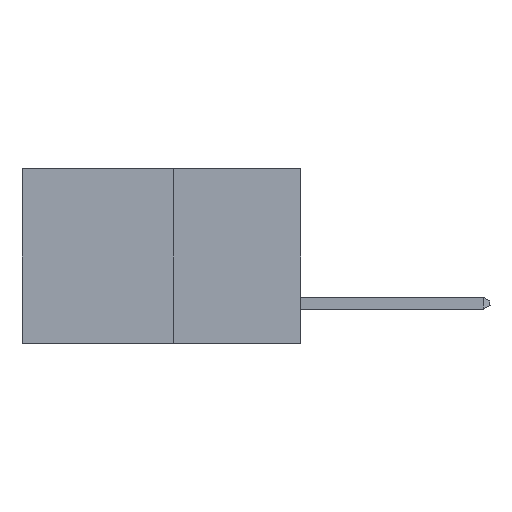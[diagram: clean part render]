
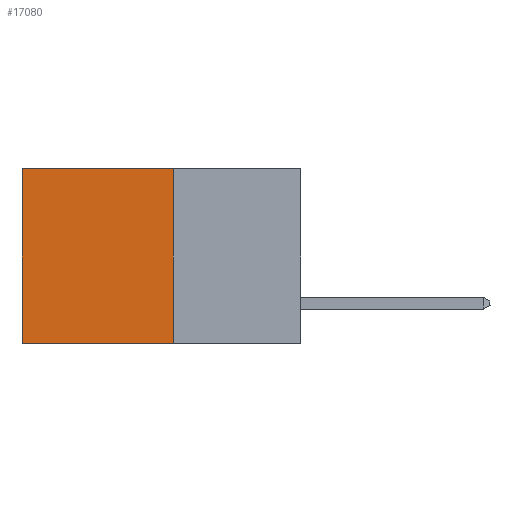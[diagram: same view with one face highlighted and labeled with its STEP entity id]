
A CAD part, left-side view. The second image highlights one B-rep face of the part: STEP entity #17080.
In plain terms, the highlighted planar face has unit normal (-1, 0, 0).
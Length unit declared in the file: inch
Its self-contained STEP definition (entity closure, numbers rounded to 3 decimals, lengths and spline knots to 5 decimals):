
#385 = VERTEX_POINT ( 'NONE', #16310 ) ;
#1076 = VECTOR ( 'NONE', #4487, 39.37008 ) ;
#3361 = VERTEX_POINT ( 'NONE', #9155 ) ;
#3442 = VECTOR ( 'NONE', #4424, 39.37008 ) ;
#3836 = CARTESIAN_POINT ( 'NONE',  ( 0.277, 0.27, -0.37 ) ) ;
#4424 = DIRECTION ( 'NONE',  ( 0., 1., 0. ) ) ;
#4487 = DIRECTION ( 'NONE',  ( 0., 1., 0. ) ) ;
#7369 = VECTOR ( 'NONE', #26057, 39.37008 ) ;
#7730 = EDGE_CURVE ( 'NONE', #3361, #16537, #18815, .T. ) ;
#8142 = DIRECTION ( 'NONE',  ( 1., 0., 0. ) ) ;
#9028 = CARTESIAN_POINT ( 'NONE',  ( 0.277, 0.59, -0.37 ) ) ;
#9155 = CARTESIAN_POINT ( 'NONE',  ( 0.277, 0.59, 0. ) ) ;
#9181 = LINE ( 'NONE', #15149, #3442 ) ;
#9739 = EDGE_LOOP ( 'NONE', ( #17895, #10420, #9876, #25412 ) ) ;
#9876 = ORIENTED_EDGE ( 'NONE', *, *, #27404, .F. ) ;
#10420 = ORIENTED_EDGE ( 'NONE', *, *, #17299, .F. ) ;
#12137 = FACE_OUTER_BOUND ( 'NONE', #9739, .T. ) ;
#12380 = PLANE ( 'NONE',  #21613 ) ;
#12692 = CARTESIAN_POINT ( 'NONE',  ( 0.277, 0.27, -0.37 ) ) ;
#15149 = CARTESIAN_POINT ( 'NONE',  ( 0.277, 0.27, 0. ) ) ;
#16310 = CARTESIAN_POINT ( 'NONE',  ( 0.277, 0.27, -0.37 ) ) ;
#16530 = EDGE_CURVE ( 'NONE', #19625, #3361, #9181, .T. ) ;
#16537 = VERTEX_POINT ( 'NONE', #21537 ) ;
#17080 = ADVANCED_FACE ( 'NONE', ( #12137 ), #12380, .F. ) ;
#17299 = EDGE_CURVE ( 'NONE', #385, #16537, #23786, .T. ) ;
#17895 = ORIENTED_EDGE ( 'NONE', *, *, #7730, .T. ) ;
#18815 = LINE ( 'NONE', #9028, #7369 ) ;
#19625 = VERTEX_POINT ( 'NONE', #26893 ) ;
#20246 = VECTOR ( 'NONE', #21259, 39.37008 ) ;
#21259 = DIRECTION ( 'NONE',  ( 0., 0., -1. ) ) ;
#21537 = CARTESIAN_POINT ( 'NONE',  ( 0.277, 0.59, -0.37 ) ) ;
#21598 = CARTESIAN_POINT ( 'NONE',  ( 0.277, 0.27, -0.37 ) ) ;
#21613 = AXIS2_PLACEMENT_3D ( 'NONE', #3836, #8142, #23084 ) ;
#23084 = DIRECTION ( 'NONE',  ( 0., 0., -1. ) ) ;
#23786 = LINE ( 'NONE', #21598, #1076 ) ;
#25412 = ORIENTED_EDGE ( 'NONE', *, *, #16530, .T. ) ;
#25852 = LINE ( 'NONE', #12692, #20246 ) ;
#26057 = DIRECTION ( 'NONE',  ( 0., 0., -1. ) ) ;
#26893 = CARTESIAN_POINT ( 'NONE',  ( 0.277, 0.27, 0. ) ) ;
#27404 = EDGE_CURVE ( 'NONE', #19625, #385, #25852, .T. ) ;
